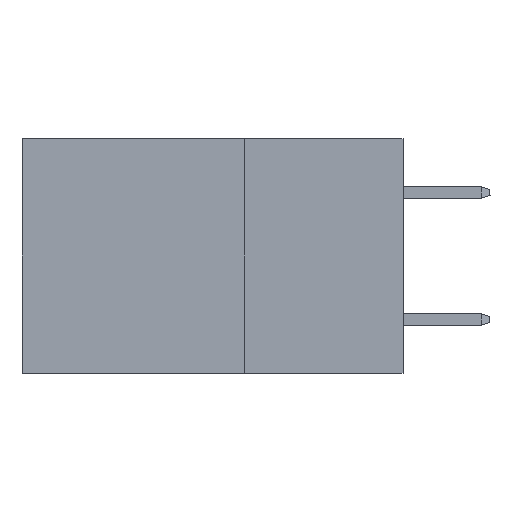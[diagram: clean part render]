
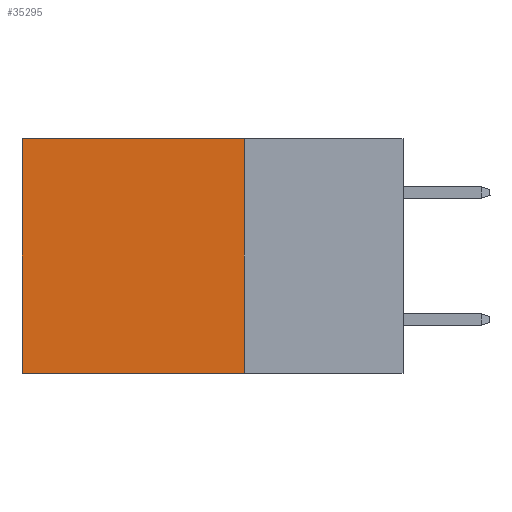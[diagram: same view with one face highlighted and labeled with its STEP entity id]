
A CAD part, left-side view. The second image highlights one B-rep face of the part: STEP entity #35295.
In plain terms, the highlighted planar face has unit normal (-1, 0, 0).
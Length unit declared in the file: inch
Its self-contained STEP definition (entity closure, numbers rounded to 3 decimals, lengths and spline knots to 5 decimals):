
#57 = VERTEX_POINT ( 'NONE', #13580 ) ;
#3310 = VECTOR ( 'NONE', #24554, 39.37008 ) ;
#5336 = DIRECTION ( 'NONE',  ( 0., 1., 0. ) ) ;
#7410 = CARTESIAN_POINT ( 'NONE',  ( 0.2875, 0.6, -0.37 ) ) ;
#7626 = VERTEX_POINT ( 'NONE', #34886 ) ;
#7777 = CARTESIAN_POINT ( 'NONE',  ( 0.2875, 0.6, 0. ) ) ;
#8447 = PLANE ( 'NONE',  #13736 ) ;
#9699 = ORIENTED_EDGE ( 'NONE', *, *, #10670, .T. ) ;
#10670 = EDGE_CURVE ( 'NONE', #7626, #12174, #35146, .T. ) ;
#12174 = VERTEX_POINT ( 'NONE', #7777 ) ;
#13580 = CARTESIAN_POINT ( 'NONE',  ( 0.2875, 0.25, -0.37 ) ) ;
#13736 = AXIS2_PLACEMENT_3D ( 'NONE', #16755, #35161, #24696 ) ;
#14231 = VECTOR ( 'NONE', #23059, 39.37008 ) ;
#15092 = CARTESIAN_POINT ( 'NONE',  ( 0.2875, 0.25, -0.37 ) ) ;
#16071 = CARTESIAN_POINT ( 'NONE',  ( 0.2875, 0.6, 0. ) ) ;
#16085 = EDGE_CURVE ( 'NONE', #57, #26324, #19958, .T. ) ;
#16755 = CARTESIAN_POINT ( 'NONE',  ( 0.2875, 0.25, 0. ) ) ;
#17019 = EDGE_CURVE ( 'NONE', #12174, #26324, #27642, .T. ) ;
#19878 = CARTESIAN_POINT ( 'NONE',  ( 0.2875, 0.25, 0. ) ) ;
#19958 = LINE ( 'NONE', #15092, #14231 ) ;
#20238 = LINE ( 'NONE', #19878, #22764 ) ;
#22764 = VECTOR ( 'NONE', #26038, 39.37008 ) ;
#23059 = DIRECTION ( 'NONE',  ( 0., 1., 0. ) ) ;
#23805 = ORIENTED_EDGE ( 'NONE', *, *, #16085, .F. ) ;
#24407 = ORIENTED_EDGE ( 'NONE', *, *, #29007, .F. ) ;
#24554 = DIRECTION ( 'NONE',  ( 0., 0., -1. ) ) ;
#24696 = DIRECTION ( 'NONE',  ( 0., 0., -1. ) ) ;
#26038 = DIRECTION ( 'NONE',  ( 0., 0., -1. ) ) ;
#26324 = VERTEX_POINT ( 'NONE', #7410 ) ;
#27426 = FACE_OUTER_BOUND ( 'NONE', #30528, .T. ) ;
#27642 = LINE ( 'NONE', #16071, #3310 ) ;
#29007 = EDGE_CURVE ( 'NONE', #7626, #57, #20238, .T. ) ;
#29668 = ORIENTED_EDGE ( 'NONE', *, *, #17019, .T. ) ;
#30528 = EDGE_LOOP ( 'NONE', ( #29668, #23805, #24407, #9699 ) ) ;
#32777 = CARTESIAN_POINT ( 'NONE',  ( 0.2875, 0.25, 0. ) ) ;
#33077 = VECTOR ( 'NONE', #5336, 39.37008 ) ;
#34886 = CARTESIAN_POINT ( 'NONE',  ( 0.2875, 0.25, 0. ) ) ;
#35146 = LINE ( 'NONE', #32777, #33077 ) ;
#35161 = DIRECTION ( 'NONE',  ( 1., 0., 0. ) ) ;
#35295 = ADVANCED_FACE ( 'NONE', ( #27426 ), #8447, .F. ) ;
